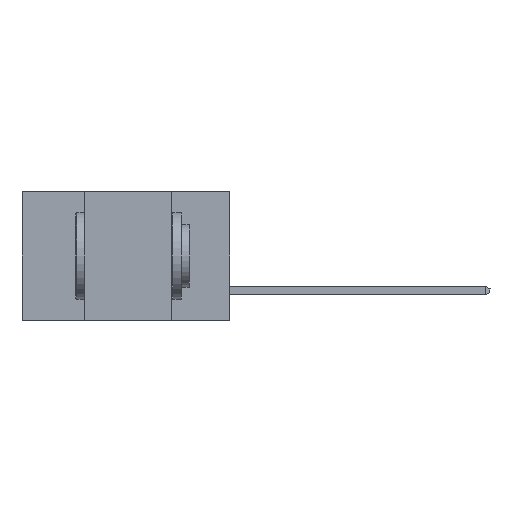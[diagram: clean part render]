
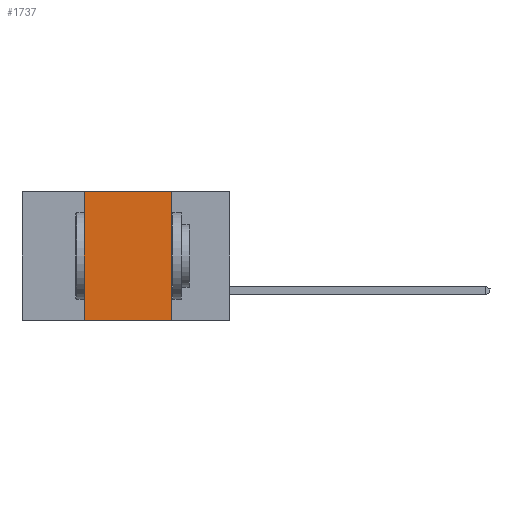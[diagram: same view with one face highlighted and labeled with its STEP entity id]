
A CAD part, left-side view. The second image highlights one B-rep face of the part: STEP entity #1737.
In plain terms, the highlighted planar face has unit normal (-1, 0, 0).
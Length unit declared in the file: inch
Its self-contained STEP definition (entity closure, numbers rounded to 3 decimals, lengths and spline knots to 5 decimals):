
#871 = EDGE_LOOP ( 'NONE', ( #14406, #1837, #6490, #17565 ) ) ;
#1225 = DIRECTION ( 'NONE',  ( 0., 0., -1. ) ) ;
#1314 = CARTESIAN_POINT ( 'NONE',  ( 0., 0.17, -0.37 ) ) ;
#1737 = ADVANCED_FACE ( 'NONE', ( #2129 ), #11955, .F. ) ;
#1837 = ORIENTED_EDGE ( 'NONE', *, *, #2802, .F. ) ;
#2129 = FACE_OUTER_BOUND ( 'NONE', #871, .T. ) ;
#2167 = VECTOR ( 'NONE', #17119, 39.37008 ) ;
#2629 = EDGE_CURVE ( 'NONE', #13797, #8262, #14713, .T. ) ;
#2784 = VECTOR ( 'NONE', #7412, 39.37008 ) ;
#2802 = EDGE_CURVE ( 'NONE', #13924, #11766, #7044, .T. ) ;
#2911 = EDGE_CURVE ( 'NONE', #13797, #13924, #10019, .T. ) ;
#3035 = AXIS2_PLACEMENT_3D ( 'NONE', #6561, #11868, #8014 ) ;
#6307 = CARTESIAN_POINT ( 'NONE',  ( 0., 0.17, -0.37 ) ) ;
#6490 = ORIENTED_EDGE ( 'NONE', *, *, #2911, .F. ) ;
#6499 = VECTOR ( 'NONE', #1225, 39.37008 ) ;
#6561 = CARTESIAN_POINT ( 'NONE',  ( 0., 0.6, 0. ) ) ;
#6873 = CARTESIAN_POINT ( 'NONE',  ( 0., 0.6, -0.37 ) ) ;
#7044 = LINE ( 'NONE', #16763, #2784 ) ;
#7412 = DIRECTION ( 'NONE',  ( 0., -1., 0. ) ) ;
#7853 = CARTESIAN_POINT ( 'NONE',  ( 0., 0.42, -0.37 ) ) ;
#8014 = DIRECTION ( 'NONE',  ( 0., 0., -1. ) ) ;
#8223 = VECTOR ( 'NONE', #17664, 39.37008 ) ;
#8262 = VERTEX_POINT ( 'NONE', #6307 ) ;
#10019 = LINE ( 'NONE', #7853, #2167 ) ;
#11766 = VERTEX_POINT ( 'NONE', #16976 ) ;
#11868 = DIRECTION ( 'NONE',  ( 1., 0., 0. ) ) ;
#11955 = PLANE ( 'NONE',  #3035 ) ;
#13669 = LINE ( 'NONE', #1314, #6499 ) ;
#13797 = VERTEX_POINT ( 'NONE', #14609 ) ;
#13924 = VERTEX_POINT ( 'NONE', #16219 ) ;
#14406 = ORIENTED_EDGE ( 'NONE', *, *, #16810, .F. ) ;
#14609 = CARTESIAN_POINT ( 'NONE',  ( 0., 0.42, -0.37 ) ) ;
#14713 = LINE ( 'NONE', #6873, #8223 ) ;
#16219 = CARTESIAN_POINT ( 'NONE',  ( 0., 0.42, 0. ) ) ;
#16763 = CARTESIAN_POINT ( 'NONE',  ( 0., 0.6, 0. ) ) ;
#16810 = EDGE_CURVE ( 'NONE', #11766, #8262, #13669, .T. ) ;
#16976 = CARTESIAN_POINT ( 'NONE',  ( 0., 0.17, 0. ) ) ;
#17119 = DIRECTION ( 'NONE',  ( 0., 0., 1. ) ) ;
#17565 = ORIENTED_EDGE ( 'NONE', *, *, #2629, .T. ) ;
#17664 = DIRECTION ( 'NONE',  ( 0., -1., 0. ) ) ;
